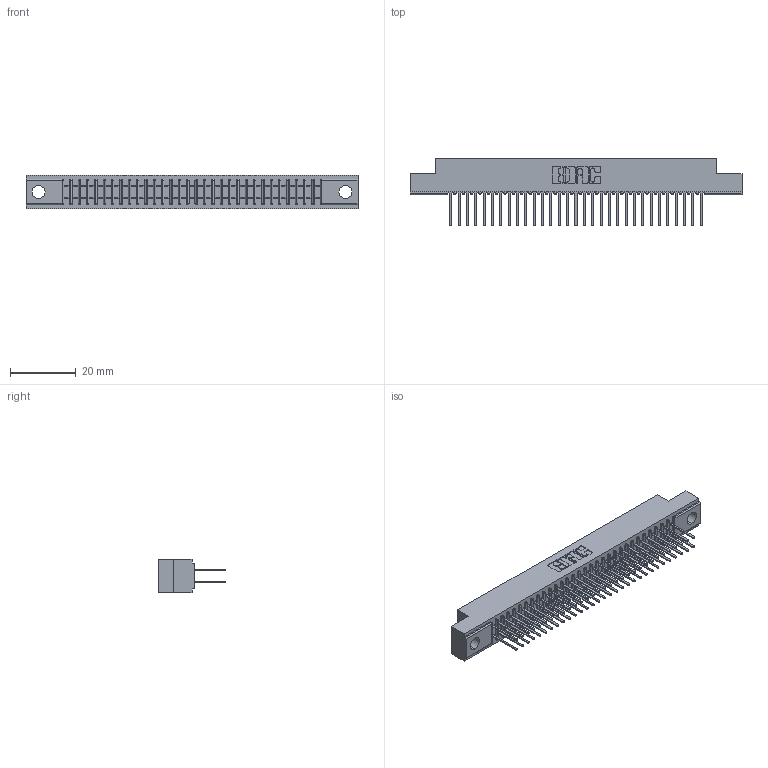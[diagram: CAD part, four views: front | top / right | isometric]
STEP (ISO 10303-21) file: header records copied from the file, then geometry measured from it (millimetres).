
FILE_DESCRIPTION (( 'STEP AP203' ), '1' );
FILE_NAME ('391-062-522-204.STEP', '2018-08-09T12:56:00', ( '' ), ( '' ), 'SwSTEP 2.0', 'SolidWorks 2016', '' );
FILE_SCHEMA (( 'CONFIG_CONTROL_DESIGN' ));
Length unit declared in the file: inch
Products named in the file (3): 341-292-001_341-292-122; 391-062-522-204; 341 Part_.156 (3.96) Dia Mounting Holes
Assembly tree (63 placements, depth 2):
  391-062-522-204
    341 Part_.156 (3.96) Dia Mounting Holes
    341-292-001_341-292-122  x62
Bounding box: 100.97 x 20.62 x 10.16 mm (x, y, z)
Volume: 7425.1 mm3; surface area: 13274.8 mm2
Topology: 63 solids, 63 shells, 4222 faces, 12225 edges, 7918 vertices
Faces by surface type: plane 2562, cylinder 1536, sphere 64, torus 60
Entity records: 39400 total; most frequent: CARTESIAN_POINT 6555, ORIENTED_EDGE 6510, DIRECTION 6361, EDGE_CURVE 3255, VECTOR 2625, LINE 2625, VERTEX_POINT 2062, AXIS2_PLACEMENT_3D 1868
